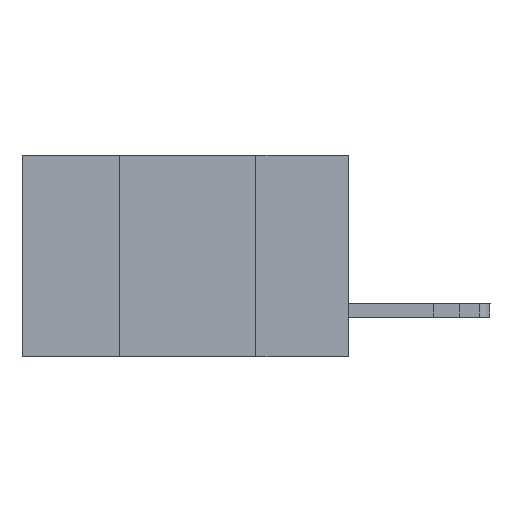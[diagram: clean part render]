
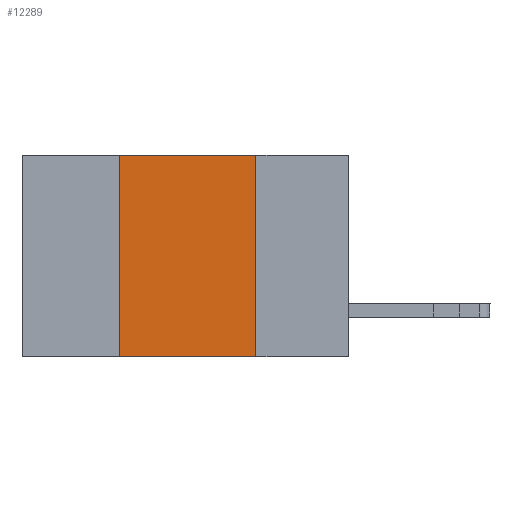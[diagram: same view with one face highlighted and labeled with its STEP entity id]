
A CAD part, left-side view. The second image highlights one B-rep face of the part: STEP entity #12289.
In plain terms, the highlighted planar face has unit normal (-1, 0, 0).
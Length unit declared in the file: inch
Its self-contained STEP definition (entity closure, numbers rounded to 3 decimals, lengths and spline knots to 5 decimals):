
#1114 = EDGE_LOOP ( 'NONE', ( #19718, #5610, #18742, #7742 ) ) ;
#1141 = CARTESIAN_POINT ( 'NONE',  ( 0., 0.42, -0.37 ) ) ;
#1590 = LINE ( 'NONE', #3996, #13371 ) ;
#3221 = PLANE ( 'NONE',  #6109 ) ;
#3996 = CARTESIAN_POINT ( 'NONE',  ( 0., 0.6, 0. ) ) ;
#4589 = VERTEX_POINT ( 'NONE', #10359 ) ;
#4920 = DIRECTION ( 'NONE',  ( 1., 0., 0. ) ) ;
#5610 = ORIENTED_EDGE ( 'NONE', *, *, #19913, .F. ) ;
#5641 = CARTESIAN_POINT ( 'NONE',  ( 0., 0.17, -0.37 ) ) ;
#5697 = DIRECTION ( 'NONE',  ( 0., -1., 0. ) ) ;
#6057 = VERTEX_POINT ( 'NONE', #16756 ) ;
#6109 = AXIS2_PLACEMENT_3D ( 'NONE', #12832, #4920, #15787 ) ;
#6626 = EDGE_CURVE ( 'NONE', #13841, #6057, #7052, .T. ) ;
#7052 = LINE ( 'NONE', #5641, #7593 ) ;
#7346 = DIRECTION ( 'NONE',  ( 0., 0., -1. ) ) ;
#7593 = VECTOR ( 'NONE', #7346, 39.37008 ) ;
#7730 = LINE ( 'NONE', #7764, #15295 ) ;
#7742 = ORIENTED_EDGE ( 'NONE', *, *, #16000, .T. ) ;
#7764 = CARTESIAN_POINT ( 'NONE',  ( 0., 0.6, -0.37 ) ) ;
#10359 = CARTESIAN_POINT ( 'NONE',  ( 0., 0.42, 0. ) ) ;
#11281 = FACE_OUTER_BOUND ( 'NONE', #1114, .T. ) ;
#11702 = CARTESIAN_POINT ( 'NONE',  ( 0., 0.17, 0. ) ) ;
#12068 = VECTOR ( 'NONE', #16889, 39.37008 ) ;
#12289 = ADVANCED_FACE ( 'NONE', ( #11281 ), #3221, .F. ) ;
#12465 = CARTESIAN_POINT ( 'NONE',  ( 0., 0.42, -0.37 ) ) ;
#12534 = LINE ( 'NONE', #1141, #12068 ) ;
#12832 = CARTESIAN_POINT ( 'NONE',  ( 0., 0.6, 0. ) ) ;
#13371 = VECTOR ( 'NONE', #5697, 39.37008 ) ;
#13841 = VERTEX_POINT ( 'NONE', #11702 ) ;
#15295 = VECTOR ( 'NONE', #16845, 39.37008 ) ;
#15787 = DIRECTION ( 'NONE',  ( 0., 0., -1. ) ) ;
#16000 = EDGE_CURVE ( 'NONE', #19165, #6057, #7730, .T. ) ;
#16756 = CARTESIAN_POINT ( 'NONE',  ( 0., 0.17, -0.37 ) ) ;
#16845 = DIRECTION ( 'NONE',  ( 0., -1., 0. ) ) ;
#16889 = DIRECTION ( 'NONE',  ( 0., 0., 1. ) ) ;
#17963 = EDGE_CURVE ( 'NONE', #19165, #4589, #12534, .T. ) ;
#18742 = ORIENTED_EDGE ( 'NONE', *, *, #17963, .F. ) ;
#19165 = VERTEX_POINT ( 'NONE', #12465 ) ;
#19718 = ORIENTED_EDGE ( 'NONE', *, *, #6626, .F. ) ;
#19913 = EDGE_CURVE ( 'NONE', #4589, #13841, #1590, .T. ) ;
